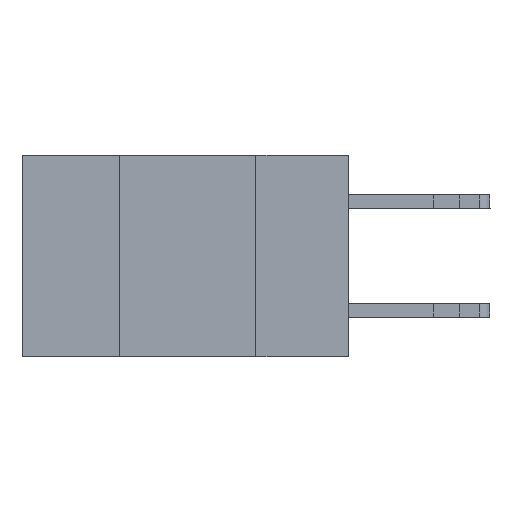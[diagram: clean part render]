
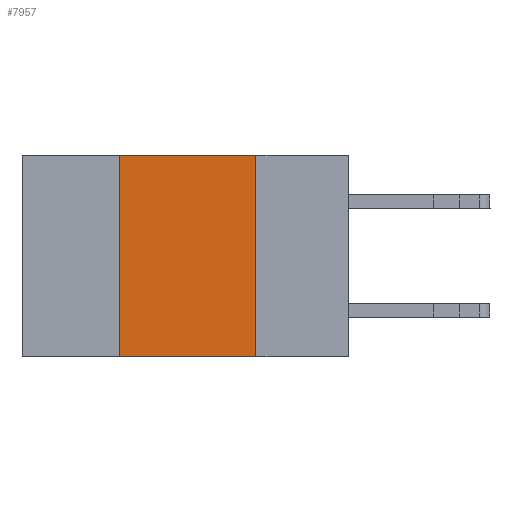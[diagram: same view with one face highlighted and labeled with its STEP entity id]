
A CAD part, left-side view. The second image highlights one B-rep face of the part: STEP entity #7957.
In plain terms, the highlighted planar face has unit normal (-1, 0, 0).
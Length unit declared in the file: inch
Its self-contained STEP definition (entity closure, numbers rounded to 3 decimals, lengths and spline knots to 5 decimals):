
#234 = CARTESIAN_POINT ( 'NONE',  ( 0., 0.42, 0. ) ) ;
#276 = CARTESIAN_POINT ( 'NONE',  ( 0., 0.17, 0. ) ) ;
#552 = EDGE_CURVE ( 'NONE', #14204, #11056, #1122, .T. ) ;
#884 = VECTOR ( 'NONE', #10244, 39.37008 ) ;
#1122 = LINE ( 'NONE', #3199, #1498 ) ;
#1133 = DIRECTION ( 'NONE',  ( 0., 0., -1. ) ) ;
#1498 = VECTOR ( 'NONE', #13655, 39.37008 ) ;
#1502 = CARTESIAN_POINT ( 'NONE',  ( 0., 0.6, 0. ) ) ;
#2038 = CARTESIAN_POINT ( 'NONE',  ( 0., 0.17, -0.37 ) ) ;
#3193 = CARTESIAN_POINT ( 'NONE',  ( 0., 0.6, -0.37 ) ) ;
#3199 = CARTESIAN_POINT ( 'NONE',  ( 0., 0.6, 0. ) ) ;
#3363 = LINE ( 'NONE', #14978, #884 ) ;
#3888 = ORIENTED_EDGE ( 'NONE', *, *, #552, .F. ) ;
#4087 = PLANE ( 'NONE',  #14022 ) ;
#4399 = LINE ( 'NONE', #3193, #12299 ) ;
#6084 = LINE ( 'NONE', #276, #12754 ) ;
#6781 = DIRECTION ( 'NONE',  ( 0., -1., 0. ) ) ;
#7140 = EDGE_CURVE ( 'NONE', #8313, #14204, #3363, .T. ) ;
#7225 = CARTESIAN_POINT ( 'NONE',  ( 0., 0.42, -0.37 ) ) ;
#7618 = DIRECTION ( 'NONE',  ( 1., 0., 0. ) ) ;
#7957 = ADVANCED_FACE ( 'NONE', ( #14560 ), #4087, .F. ) ;
#8313 = VERTEX_POINT ( 'NONE', #7225 ) ;
#8869 = ORIENTED_EDGE ( 'NONE', *, *, #9068, .F. ) ;
#9068 = EDGE_CURVE ( 'NONE', #11056, #9348, #6084, .T. ) ;
#9348 = VERTEX_POINT ( 'NONE', #2038 ) ;
#9745 = ORIENTED_EDGE ( 'NONE', *, *, #7140, .F. ) ;
#9807 = CARTESIAN_POINT ( 'NONE',  ( 0., 0.17, 0. ) ) ;
#10244 = DIRECTION ( 'NONE',  ( 0., 0., 1. ) ) ;
#10342 = EDGE_CURVE ( 'NONE', #8313, #9348, #4399, .T. ) ;
#11056 = VERTEX_POINT ( 'NONE', #9807 ) ;
#11919 = EDGE_LOOP ( 'NONE', ( #8869, #3888, #9745, #14708 ) ) ;
#12299 = VECTOR ( 'NONE', #6781, 39.37008 ) ;
#12576 = DIRECTION ( 'NONE',  ( 0., 0., -1. ) ) ;
#12754 = VECTOR ( 'NONE', #1133, 39.37008 ) ;
#13655 = DIRECTION ( 'NONE',  ( 0., -1., 0. ) ) ;
#14022 = AXIS2_PLACEMENT_3D ( 'NONE', #1502, #7618, #12576 ) ;
#14204 = VERTEX_POINT ( 'NONE', #234 ) ;
#14560 = FACE_OUTER_BOUND ( 'NONE', #11919, .T. ) ;
#14708 = ORIENTED_EDGE ( 'NONE', *, *, #10342, .T. ) ;
#14978 = CARTESIAN_POINT ( 'NONE',  ( 0., 0.42, 0. ) ) ;
